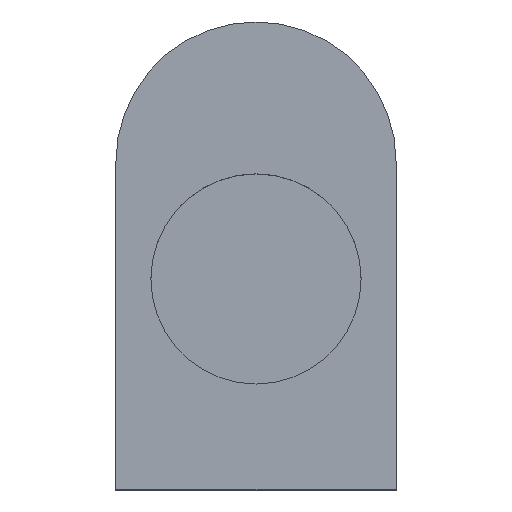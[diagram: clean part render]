
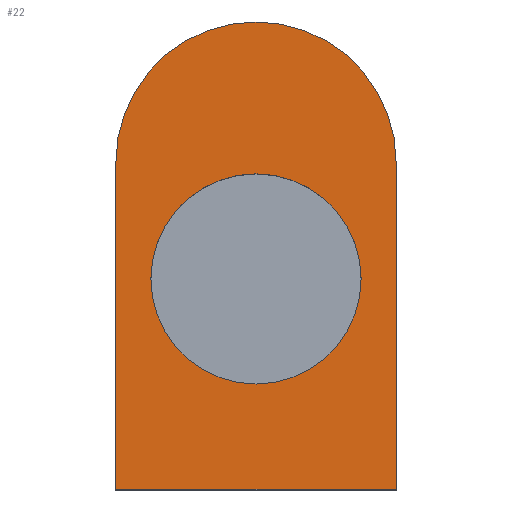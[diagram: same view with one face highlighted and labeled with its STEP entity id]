
A CAD part, top view. The second image highlights one B-rep face of the part: STEP entity #22.
In plain terms, the highlighted planar face has unit normal (0, 0, 1).
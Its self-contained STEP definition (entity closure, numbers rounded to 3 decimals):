
#20 = AXIS2_PLACEMENT_3D ( 'NONE', #64, #159, #345 ) ;
#22 = ADVANCED_FACE ( 'NONE', ( #306, #134 ), #224, .T. ) ;
#34 = VERTEX_POINT ( 'NONE', #260 ) ;
#38 = ORIENTED_EDGE ( 'NONE', *, *, #196, .T. ) ;
#64 = CARTESIAN_POINT ( 'NONE',  ( 0., -5., 40. ) ) ;
#73 = AXIS2_PLACEMENT_3D ( 'NONE', #550, #414, #101 ) ;
#85 = CARTESIAN_POINT ( 'NONE',  ( 6., -14., 40. ) ) ;
#88 = EDGE_CURVE ( 'NONE', #512, #471, #417, .T. ) ;
#95 = CIRCLE ( 'NONE', #20, 4.5 ) ;
#101 = DIRECTION ( 'NONE',  ( 1., 0., 0. ) ) ;
#105 = AXIS2_PLACEMENT_3D ( 'NONE', #488, #176, #493 ) ;
#107 = ORIENTED_EDGE ( 'NONE', *, *, #303, .T. ) ;
#131 = EDGE_CURVE ( 'NONE', #211, #34, #289, .T. ) ;
#134 = FACE_OUTER_BOUND ( 'NONE', #257, .T. ) ;
#144 = ORIENTED_EDGE ( 'NONE', *, *, #503, .T. ) ;
#155 = CARTESIAN_POINT ( 'NONE',  ( -6., 0., 40. ) ) ;
#159 = DIRECTION ( 'NONE',  ( 0., 0., -1. ) ) ;
#163 = VECTOR ( 'NONE', #179, 1000. ) ;
#176 = DIRECTION ( 'NONE',  ( 0., 0., 1. ) ) ;
#179 = DIRECTION ( 'NONE',  ( 0., 1., 0. ) ) ;
#192 = CARTESIAN_POINT ( 'NONE',  ( -6., 0., 40. ) ) ;
#196 = EDGE_CURVE ( 'NONE', #471, #211, #315, .T. ) ;
#198 = VERTEX_POINT ( 'NONE', #259 ) ;
#211 = VERTEX_POINT ( 'NONE', #85 ) ;
#224 = PLANE ( 'NONE',  #105 ) ;
#225 = CIRCLE ( 'NONE', #524, 4.5 ) ;
#239 = CIRCLE ( 'NONE', #73, 6. ) ;
#257 = EDGE_LOOP ( 'NONE', ( #514, #373, #38, #426 ) ) ;
#259 = CARTESIAN_POINT ( 'NONE',  ( 4.5, -5., 40. ) ) ;
#260 = CARTESIAN_POINT ( 'NONE',  ( 6., 0., 40. ) ) ;
#289 = LINE ( 'NONE', #505, #163 ) ;
#303 = EDGE_CURVE ( 'NONE', #198, #518, #225, .T. ) ;
#305 = DIRECTION ( 'NONE',  ( 1., 0., 0. ) ) ;
#306 = FACE_BOUND ( 'NONE', #379, .T. ) ;
#315 = LINE ( 'NONE', #535, #347 ) ;
#345 = DIRECTION ( 'NONE',  ( 1., 0., 0. ) ) ;
#347 = VECTOR ( 'NONE', #305, 1000. ) ;
#351 = DIRECTION ( 'NONE',  ( 1., 0., 0. ) ) ;
#373 = ORIENTED_EDGE ( 'NONE', *, *, #88, .T. ) ;
#379 = EDGE_LOOP ( 'NONE', ( #144, #107 ) ) ;
#387 = CARTESIAN_POINT ( 'NONE',  ( -6., -14., 40. ) ) ;
#397 = EDGE_CURVE ( 'NONE', #34, #512, #239, .T. ) ;
#414 = DIRECTION ( 'NONE',  ( 0., 0., 1. ) ) ;
#417 = LINE ( 'NONE', #192, #567 ) ;
#426 = ORIENTED_EDGE ( 'NONE', *, *, #131, .T. ) ;
#454 = CARTESIAN_POINT ( 'NONE',  ( 0., -5., 40. ) ) ;
#471 = VERTEX_POINT ( 'NONE', #387 ) ;
#488 = CARTESIAN_POINT ( 'NONE',  ( 0., 0., 40. ) ) ;
#493 = DIRECTION ( 'NONE',  ( 1., 0., 0. ) ) ;
#503 = EDGE_CURVE ( 'NONE', #518, #198, #95, .T. ) ;
#505 = CARTESIAN_POINT ( 'NONE',  ( 6., -14., 40. ) ) ;
#511 = DIRECTION ( 'NONE',  ( 0., -1., 0. ) ) ;
#512 = VERTEX_POINT ( 'NONE', #155 ) ;
#514 = ORIENTED_EDGE ( 'NONE', *, *, #397, .T. ) ;
#518 = VERTEX_POINT ( 'NONE', #564 ) ;
#524 = AXIS2_PLACEMENT_3D ( 'NONE', #454, #568, #351 ) ;
#535 = CARTESIAN_POINT ( 'NONE',  ( -6., -14., 40. ) ) ;
#550 = CARTESIAN_POINT ( 'NONE',  ( 0., 0., 40. ) ) ;
#564 = CARTESIAN_POINT ( 'NONE',  ( -4.5, -5., 40. ) ) ;
#567 = VECTOR ( 'NONE', #511, 1000. ) ;
#568 = DIRECTION ( 'NONE',  ( 0., 0., -1. ) ) ;
